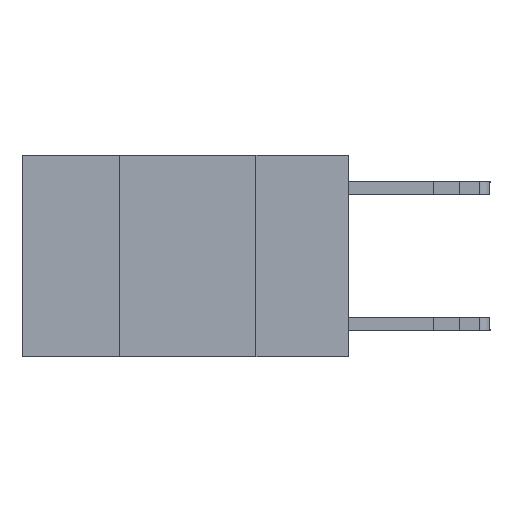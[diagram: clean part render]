
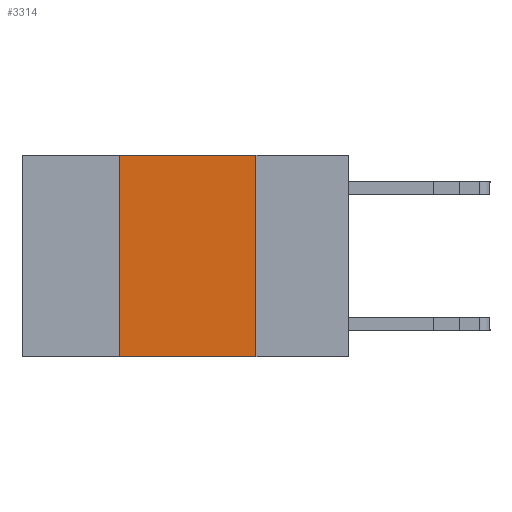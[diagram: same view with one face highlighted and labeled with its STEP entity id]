
A CAD part, left-side view. The second image highlights one B-rep face of the part: STEP entity #3314.
In plain terms, the highlighted planar face has unit normal (-1, 0, 0).
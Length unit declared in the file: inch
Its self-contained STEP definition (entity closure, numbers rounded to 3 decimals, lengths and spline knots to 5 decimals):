
#144 = VERTEX_POINT ( 'NONE', #1016 ) ;
#1016 = CARTESIAN_POINT ( 'NONE',  ( 0., 0.17, -0.37 ) ) ;
#1170 = FACE_OUTER_BOUND ( 'NONE', #3005, .T. ) ;
#1298 = LINE ( 'NONE', #18633, #16521 ) ;
#1486 = EDGE_CURVE ( 'NONE', #12539, #144, #1298, .T. ) ;
#2610 = ORIENTED_EDGE ( 'NONE', *, *, #15652, .F. ) ;
#3005 = EDGE_LOOP ( 'NONE', ( #10798, #12975, #2610, #15493 ) ) ;
#3314 = ADVANCED_FACE ( 'NONE', ( #1170 ), #17692, .F. ) ;
#4177 = DIRECTION ( 'NONE',  ( 0., 0., -1. ) ) ;
#4727 = VERTEX_POINT ( 'NONE', #16431 ) ;
#4761 = LINE ( 'NONE', #12310, #10637 ) ;
#7457 = EDGE_CURVE ( 'NONE', #4727, #12539, #4761, .T. ) ;
#9633 = CARTESIAN_POINT ( 'NONE',  ( 0., 0.17, 0. ) ) ;
#10460 = DIRECTION ( 'NONE',  ( 0., -1., 0. ) ) ;
#10637 = VECTOR ( 'NONE', #10460, 39.37008 ) ;
#10784 = LINE ( 'NONE', #15172, #15102 ) ;
#10798 = ORIENTED_EDGE ( 'NONE', *, *, #1486, .F. ) ;
#11585 = CARTESIAN_POINT ( 'NONE',  ( 0., 0.6, 0. ) ) ;
#12310 = CARTESIAN_POINT ( 'NONE',  ( 0., 0.6, 0. ) ) ;
#12539 = VERTEX_POINT ( 'NONE', #9633 ) ;
#12975 = ORIENTED_EDGE ( 'NONE', *, *, #7457, .F. ) ;
#13045 = CARTESIAN_POINT ( 'NONE',  ( 0., 0.42, 0. ) ) ;
#13160 = AXIS2_PLACEMENT_3D ( 'NONE', #11585, #15767, #18968 ) ;
#13944 = VERTEX_POINT ( 'NONE', #16454 ) ;
#15102 = VECTOR ( 'NONE', #15355, 39.37008 ) ;
#15172 = CARTESIAN_POINT ( 'NONE',  ( 0., 0.6, -0.37 ) ) ;
#15355 = DIRECTION ( 'NONE',  ( 0., -1., 0. ) ) ;
#15493 = ORIENTED_EDGE ( 'NONE', *, *, #16459, .T. ) ;
#15652 = EDGE_CURVE ( 'NONE', #13944, #4727, #19073, .T. ) ;
#15766 = DIRECTION ( 'NONE',  ( 0., 0., 1. ) ) ;
#15767 = DIRECTION ( 'NONE',  ( 1., 0., 0. ) ) ;
#16431 = CARTESIAN_POINT ( 'NONE',  ( 0., 0.42, 0. ) ) ;
#16454 = CARTESIAN_POINT ( 'NONE',  ( 0., 0.42, -0.37 ) ) ;
#16459 = EDGE_CURVE ( 'NONE', #13944, #144, #10784, .T. ) ;
#16521 = VECTOR ( 'NONE', #4177, 39.37008 ) ;
#16922 = VECTOR ( 'NONE', #15766, 39.37008 ) ;
#17692 = PLANE ( 'NONE',  #13160 ) ;
#18633 = CARTESIAN_POINT ( 'NONE',  ( 0., 0.17, 0. ) ) ;
#18968 = DIRECTION ( 'NONE',  ( 0., 0., -1. ) ) ;
#19073 = LINE ( 'NONE', #13045, #16922 ) ;
